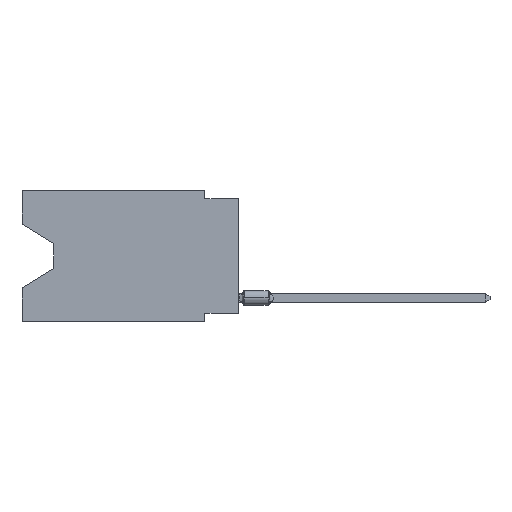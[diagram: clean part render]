
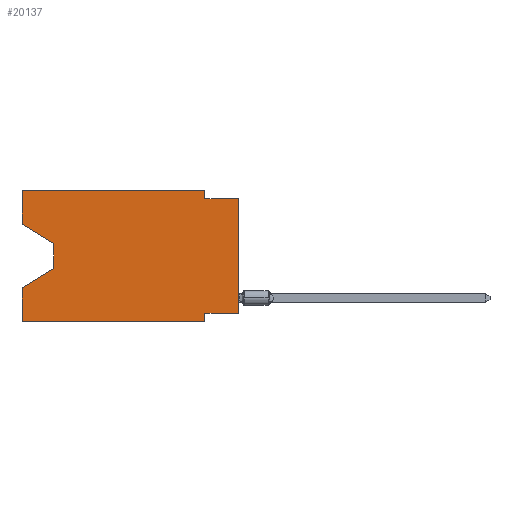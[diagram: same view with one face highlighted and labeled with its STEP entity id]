
A CAD part, left-side view. The second image highlights one B-rep face of the part: STEP entity #20137.
In plain terms, the highlighted planar face has unit normal (-1, 0, 0).
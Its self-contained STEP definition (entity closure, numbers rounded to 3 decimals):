
#268 = EDGE_CURVE ( 'NONE', #2938, #19395, #10697, .T. ) ;
#347 = LINE ( 'NONE', #9887, #1833 ) ;
#396 = FACE_OUTER_BOUND ( 'NONE', #11575, .T. ) ;
#427 = DIRECTION ( 'NONE',  ( 0., 0., 1. ) ) ;
#573 = ORIENTED_EDGE ( 'NONE', *, *, #12195, .F. ) ;
#619 = AXIS2_PLACEMENT_3D ( 'NONE', #24017, #6119, #8144 ) ;
#750 = VERTEX_POINT ( 'NONE', #24002 ) ;
#807 = VERTEX_POINT ( 'NONE', #21044 ) ;
#931 = LINE ( 'NONE', #6904, #21680 ) ;
#1037 = CARTESIAN_POINT ( 'NONE',  ( 0., 2.54, -9.271 ) ) ;
#1833 = VECTOR ( 'NONE', #4158, 1000. ) ;
#1977 = LINE ( 'NONE', #11881, #21961 ) ;
#1993 = LINE ( 'NONE', #24524, #2636 ) ;
#2636 = VECTOR ( 'NONE', #10806, 1000. ) ;
#2933 = CARTESIAN_POINT ( 'NONE',  ( 0., 2.54, -9.906 ) ) ;
#2938 = VERTEX_POINT ( 'NONE', #1037 ) ;
#3807 = CARTESIAN_POINT ( 'NONE',  ( 0., 0., -0.635 ) ) ;
#3889 = CARTESIAN_POINT ( 'NONE',  ( 0., 0., 0. ) ) ;
#4158 = DIRECTION ( 'NONE',  ( 0., -1., 0. ) ) ;
#4173 = ORIENTED_EDGE ( 'NONE', *, *, #10920, .F. ) ;
#4834 = CARTESIAN_POINT ( 'NONE',  ( 0., 16.383, -2.546 ) ) ;
#4883 = EDGE_CURVE ( 'NONE', #18654, #6125, #347, .T. ) ;
#4966 = DIRECTION ( 'NONE',  ( 0., 0., -1. ) ) ;
#4981 = CARTESIAN_POINT ( 'NONE',  ( 0., 16.383, -2.546 ) ) ;
#5060 = CARTESIAN_POINT ( 'NONE',  ( 0., 13.97, -4.013 ) ) ;
#5385 = ORIENTED_EDGE ( 'NONE', *, *, #9013, .F. ) ;
#5613 = CARTESIAN_POINT ( 'NONE',  ( 0., 13.97, -5.893 ) ) ;
#6119 = DIRECTION ( 'NONE',  ( 1., 0., 0. ) ) ;
#6125 = VERTEX_POINT ( 'NONE', #3807 ) ;
#6536 = EDGE_CURVE ( 'NONE', #17074, #807, #1977, .T. ) ;
#6904 = CARTESIAN_POINT ( 'NONE',  ( 0., 13.97, -5.893 ) ) ;
#7464 = VECTOR ( 'NONE', #16431, 1000. ) ;
#7751 = VERTEX_POINT ( 'NONE', #16156 ) ;
#7812 = ORIENTED_EDGE ( 'NONE', *, *, #16856, .F. ) ;
#7960 = VERTEX_POINT ( 'NONE', #4834 ) ;
#8144 = DIRECTION ( 'NONE',  ( 0., 0., -1. ) ) ;
#8326 = CARTESIAN_POINT ( 'NONE',  ( 0., 16.383, -9.906 ) ) ;
#8331 = ORIENTED_EDGE ( 'NONE', *, *, #8937, .T. ) ;
#8549 = ORIENTED_EDGE ( 'NONE', *, *, #4883, .F. ) ;
#8561 = VECTOR ( 'NONE', #17573, 1000. ) ;
#8585 = ORIENTED_EDGE ( 'NONE', *, *, #11265, .T. ) ;
#8742 = VECTOR ( 'NONE', #4966, 1000. ) ;
#8828 = DIRECTION ( 'NONE',  ( 0., 0.855, -0.519 ) ) ;
#8937 = EDGE_CURVE ( 'NONE', #7751, #18732, #10408, .T. ) ;
#9013 = EDGE_CURVE ( 'NONE', #7960, #22346, #14200, .T. ) ;
#9131 = EDGE_CURVE ( 'NONE', #7960, #7751, #18696, .T. ) ;
#9830 = CARTESIAN_POINT ( 'NONE',  ( 0., 16.383, 0. ) ) ;
#9887 = CARTESIAN_POINT ( 'NONE',  ( 0., 0., -0.635 ) ) ;
#10110 = LINE ( 'NONE', #3889, #16883 ) ;
#10112 = LINE ( 'NONE', #8326, #24947 ) ;
#10278 = CARTESIAN_POINT ( 'NONE',  ( 0., 0., -9.271 ) ) ;
#10408 = LINE ( 'NONE', #5060, #22059 ) ;
#10697 = LINE ( 'NONE', #2933, #8742 ) ;
#10715 = VECTOR ( 'NONE', #22085, 1000. ) ;
#10806 = DIRECTION ( 'NONE',  ( 0., 0., -1. ) ) ;
#10920 = EDGE_CURVE ( 'NONE', #22346, #14452, #20118, .T. ) ;
#11098 = EDGE_CURVE ( 'NONE', #17074, #19395, #10112, .T. ) ;
#11265 = EDGE_CURVE ( 'NONE', #18732, #807, #931, .T. ) ;
#11285 = ORIENTED_EDGE ( 'NONE', *, *, #6536, .F. ) ;
#11575 = EDGE_LOOP ( 'NONE', ( #19740, #8331, #8585, #11285, #17073, #15791, #7812, #15275, #8549, #573, #4173, #5385 ) ) ;
#11881 = CARTESIAN_POINT ( 'NONE',  ( 0., 16.383, 0. ) ) ;
#12195 = EDGE_CURVE ( 'NONE', #14452, #18654, #1993, .T. ) ;
#12562 = DIRECTION ( 'NONE',  ( 0., 0., 1. ) ) ;
#14200 = LINE ( 'NONE', #21948, #14353 ) ;
#14333 = LINE ( 'NONE', #10278, #10715 ) ;
#14353 = VECTOR ( 'NONE', #12562, 1000. ) ;
#14452 = VERTEX_POINT ( 'NONE', #20697 ) ;
#15275 = ORIENTED_EDGE ( 'NONE', *, *, #22833, .T. ) ;
#15458 = CARTESIAN_POINT ( 'NONE',  ( 0., 16.383, -9.906 ) ) ;
#15791 = ORIENTED_EDGE ( 'NONE', *, *, #268, .F. ) ;
#16156 = CARTESIAN_POINT ( 'NONE',  ( 0., 13.97, -4.013 ) ) ;
#16267 = PLANE ( 'NONE',  #619 ) ;
#16431 = DIRECTION ( 'NONE',  ( 0., -0.855, -0.519 ) ) ;
#16856 = EDGE_CURVE ( 'NONE', #750, #2938, #14333, .T. ) ;
#16883 = VECTOR ( 'NONE', #23467, 1000. ) ;
#17073 = ORIENTED_EDGE ( 'NONE', *, *, #11098, .T. ) ;
#17074 = VERTEX_POINT ( 'NONE', #15458 ) ;
#17085 = CARTESIAN_POINT ( 'NONE',  ( 0., 16.383, 0. ) ) ;
#17573 = DIRECTION ( 'NONE',  ( 0., -1., 0. ) ) ;
#18316 = CARTESIAN_POINT ( 'NONE',  ( 0., 2.54, -0.635 ) ) ;
#18392 = DIRECTION ( 'NONE',  ( 0., 0., -1. ) ) ;
#18654 = VERTEX_POINT ( 'NONE', #18316 ) ;
#18696 = LINE ( 'NONE', #4981, #7464 ) ;
#18732 = VERTEX_POINT ( 'NONE', #5613 ) ;
#19395 = VERTEX_POINT ( 'NONE', #24227 ) ;
#19740 = ORIENTED_EDGE ( 'NONE', *, *, #9131, .T. ) ;
#19886 = DIRECTION ( 'NONE',  ( 0., -1., 0. ) ) ;
#20118 = LINE ( 'NONE', #9830, #8561 ) ;
#20137 = ADVANCED_FACE ( 'NONE', ( #396 ), #16267, .F. ) ;
#20697 = CARTESIAN_POINT ( 'NONE',  ( 0., 2.54, 0. ) ) ;
#21044 = CARTESIAN_POINT ( 'NONE',  ( 0., 16.383, -7.36 ) ) ;
#21680 = VECTOR ( 'NONE', #8828, 1000. ) ;
#21948 = CARTESIAN_POINT ( 'NONE',  ( 0., 16.383, 0. ) ) ;
#21961 = VECTOR ( 'NONE', #427, 1000. ) ;
#22059 = VECTOR ( 'NONE', #18392, 1000. ) ;
#22085 = DIRECTION ( 'NONE',  ( 0., 1., 0. ) ) ;
#22346 = VERTEX_POINT ( 'NONE', #17085 ) ;
#22833 = EDGE_CURVE ( 'NONE', #750, #6125, #10110, .T. ) ;
#23467 = DIRECTION ( 'NONE',  ( 0., 0., 1. ) ) ;
#24002 = CARTESIAN_POINT ( 'NONE',  ( 0., 0., -9.271 ) ) ;
#24017 = CARTESIAN_POINT ( 'NONE',  ( 0., 16.383, 0. ) ) ;
#24227 = CARTESIAN_POINT ( 'NONE',  ( 0., 2.54, -9.906 ) ) ;
#24524 = CARTESIAN_POINT ( 'NONE',  ( 0., 2.54, 0. ) ) ;
#24947 = VECTOR ( 'NONE', #19886, 1000. ) ;
